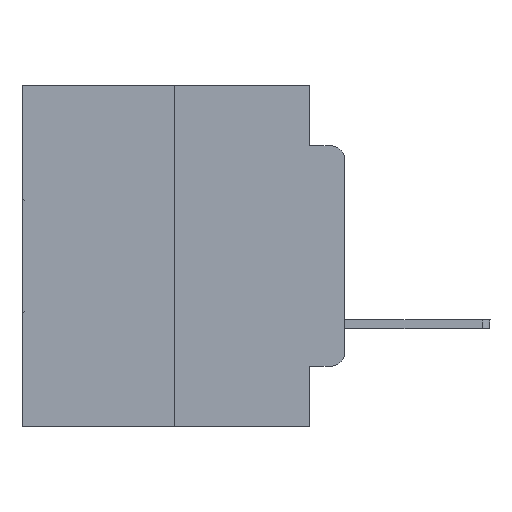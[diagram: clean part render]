
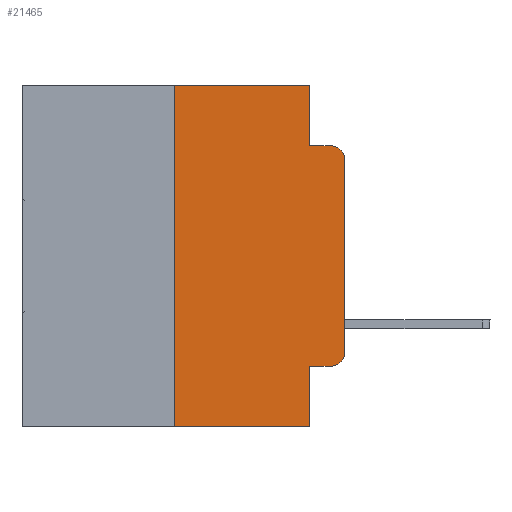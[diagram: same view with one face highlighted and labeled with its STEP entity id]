
A CAD part, left-side view. The second image highlights one B-rep face of the part: STEP entity #21465.
In plain terms, the highlighted planar face has unit normal (-1, 0, 0).
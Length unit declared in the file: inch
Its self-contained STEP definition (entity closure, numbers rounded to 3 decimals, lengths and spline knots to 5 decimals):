
#18 = LINE ( 'NONE', #8646, #12832 ) ;
#384 = CARTESIAN_POINT ( 'NONE',  ( 0., 0.25, -0.5 ) ) ;
#509 = VERTEX_POINT ( 'NONE', #1421 ) ;
#519 = EDGE_CURVE ( 'NONE', #12336, #18329, #22725, .T. ) ;
#858 = ORIENTED_EDGE ( 'NONE', *, *, #20175, .T. ) ;
#1063 = DIRECTION ( 'NONE',  ( -1., 0., 0. ) ) ;
#1421 = CARTESIAN_POINT ( 'NONE',  ( 0., 0.25, 0. ) ) ;
#1689 = VECTOR ( 'NONE', #12039, 39.37008 ) ;
#2119 = EDGE_CURVE ( 'NONE', #12896, #6646, #10922, .T. ) ;
#2352 = VECTOR ( 'NONE', #19069, 39.37008 ) ;
#2732 = CARTESIAN_POINT ( 'NONE',  ( 0., 0.051, -0.4115 ) ) ;
#3836 = VERTEX_POINT ( 'NONE', #13473 ) ;
#4869 = LINE ( 'NONE', #22501, #25134 ) ;
#5114 = AXIS2_PLACEMENT_3D ( 'NONE', #24901, #14475, #14336 ) ;
#5531 = VECTOR ( 'NONE', #14047, 39.37008 ) ;
#5994 = ORIENTED_EDGE ( 'NONE', *, *, #22789, .T. ) ;
#6082 = DIRECTION ( 'NONE',  ( 0., 0., -1. ) ) ;
#6646 = VERTEX_POINT ( 'NONE', #12520 ) ;
#6706 = DIRECTION ( 'NONE',  ( 0., 0., 1. ) ) ;
#7362 = EDGE_CURVE ( 'NONE', #26900, #12896, #23975, .T. ) ;
#7705 = PLANE ( 'NONE',  #5114 ) ;
#7989 = DIRECTION ( 'NONE',  ( 0., 0., -1. ) ) ;
#8122 = EDGE_CURVE ( 'NONE', #6646, #16722, #8678, .T. ) ;
#8245 = AXIS2_PLACEMENT_3D ( 'NONE', #20702, #1063, #7989 ) ;
#8646 = CARTESIAN_POINT ( 'NONE',  ( 0., 0.473, -0.5 ) ) ;
#8678 = CIRCLE ( 'NONE', #8245, 0.02 ) ;
#8717 = VERTEX_POINT ( 'NONE', #13815 ) ;
#9290 = CARTESIAN_POINT ( 'NONE',  ( 0., 0.051, -0.5 ) ) ;
#9889 = DIRECTION ( 'NONE',  ( -1., 0., 0. ) ) ;
#10617 = ORIENTED_EDGE ( 'NONE', *, *, #2119, .T. ) ;
#10922 = LINE ( 'NONE', #13599, #22407 ) ;
#11024 = DIRECTION ( 'NONE',  ( 0., -1., 0. ) ) ;
#11562 = ORIENTED_EDGE ( 'NONE', *, *, #14451, .F. ) ;
#11767 = CARTESIAN_POINT ( 'NONE',  ( 0., 0.25, 0. ) ) ;
#11982 = CARTESIAN_POINT ( 'NONE',  ( 0., 0.02, -0.0885 ) ) ;
#12039 = DIRECTION ( 'NONE',  ( 0., 0., 1. ) ) ;
#12336 = VERTEX_POINT ( 'NONE', #2732 ) ;
#12520 = CARTESIAN_POINT ( 'NONE',  ( 0., 0., -0.1085 ) ) ;
#12832 = VECTOR ( 'NONE', #19106, 39.37008 ) ;
#12896 = VERTEX_POINT ( 'NONE', #20054 ) ;
#13170 = AXIS2_PLACEMENT_3D ( 'NONE', #25533, #9889, #6082 ) ;
#13473 = CARTESIAN_POINT ( 'NONE',  ( 0., 0.051, -0.0885 ) ) ;
#13599 = CARTESIAN_POINT ( 'NONE',  ( 0., 0., 0. ) ) ;
#13815 = CARTESIAN_POINT ( 'NONE',  ( 0., 0.051, 0. ) ) ;
#14047 = DIRECTION ( 'NONE',  ( 0., -1., 0. ) ) ;
#14336 = DIRECTION ( 'NONE',  ( 0., 0., -1. ) ) ;
#14403 = DIRECTION ( 'NONE',  ( 0., -1., 0. ) ) ;
#14451 = EDGE_CURVE ( 'NONE', #8717, #3836, #4869, .T. ) ;
#14475 = DIRECTION ( 'NONE',  ( 1., 0., 0. ) ) ;
#14545 = EDGE_CURVE ( 'NONE', #15682, #509, #18138, .T. ) ;
#14992 = ORIENTED_EDGE ( 'NONE', *, *, #14545, .F. ) ;
#15008 = VECTOR ( 'NONE', #11024, 39.37008 ) ;
#15467 = DIRECTION ( 'NONE',  ( 0., 0., -1. ) ) ;
#15538 = ORIENTED_EDGE ( 'NONE', *, *, #8122, .T. ) ;
#15682 = VERTEX_POINT ( 'NONE', #384 ) ;
#16313 = LINE ( 'NONE', #24895, #5531 ) ;
#16662 = LINE ( 'NONE', #20617, #27791 ) ;
#16722 = VERTEX_POINT ( 'NONE', #11982 ) ;
#17001 = ORIENTED_EDGE ( 'NONE', *, *, #7362, .T. ) ;
#17274 = ORIENTED_EDGE ( 'NONE', *, *, #19019, .F. ) ;
#17455 = EDGE_LOOP ( 'NONE', ( #10617, #15538, #17274, #11562, #22049, #14992, #5994, #24530, #858, #17001 ) ) ;
#17665 = LINE ( 'NONE', #26240, #15008 ) ;
#18138 = LINE ( 'NONE', #11767, #1689 ) ;
#18329 = VERTEX_POINT ( 'NONE', #9290 ) ;
#19019 = EDGE_CURVE ( 'NONE', #3836, #16722, #17665, .T. ) ;
#19069 = DIRECTION ( 'NONE',  ( 0., 0., -1. ) ) ;
#19106 = DIRECTION ( 'NONE',  ( 0., -1., 0. ) ) ;
#20054 = CARTESIAN_POINT ( 'NONE',  ( 0., 0., -0.3915 ) ) ;
#20175 = EDGE_CURVE ( 'NONE', #12336, #26900, #16313, .T. ) ;
#20617 = CARTESIAN_POINT ( 'NONE',  ( 0., 0.473, 0. ) ) ;
#20702 = CARTESIAN_POINT ( 'NONE',  ( 0., 0.02, -0.1085 ) ) ;
#21096 = CARTESIAN_POINT ( 'NONE',  ( 0., 0.02, -0.4115 ) ) ;
#21465 = ADVANCED_FACE ( 'NONE', ( #27018 ), #7705, .F. ) ;
#22049 = ORIENTED_EDGE ( 'NONE', *, *, #26076, .F. ) ;
#22407 = VECTOR ( 'NONE', #6706, 39.37008 ) ;
#22501 = CARTESIAN_POINT ( 'NONE',  ( 0., 0.051, 0. ) ) ;
#22725 = LINE ( 'NONE', #22867, #2352 ) ;
#22789 = EDGE_CURVE ( 'NONE', #15682, #18329, #18, .T. ) ;
#22867 = CARTESIAN_POINT ( 'NONE',  ( 0., 0.051, 0. ) ) ;
#23975 = CIRCLE ( 'NONE', #13170, 0.02 ) ;
#24530 = ORIENTED_EDGE ( 'NONE', *, *, #519, .F. ) ;
#24895 = CARTESIAN_POINT ( 'NONE',  ( 0., 0.051, -0.4115 ) ) ;
#24901 = CARTESIAN_POINT ( 'NONE',  ( 0., 0.473, 0. ) ) ;
#25134 = VECTOR ( 'NONE', #15467, 39.37008 ) ;
#25533 = CARTESIAN_POINT ( 'NONE',  ( 0., 0.02, -0.3915 ) ) ;
#26076 = EDGE_CURVE ( 'NONE', #509, #8717, #16662, .T. ) ;
#26240 = CARTESIAN_POINT ( 'NONE',  ( 0., 0.051, -0.0885 ) ) ;
#26900 = VERTEX_POINT ( 'NONE', #21096 ) ;
#27018 = FACE_OUTER_BOUND ( 'NONE', #17455, .T. ) ;
#27791 = VECTOR ( 'NONE', #14403, 39.37008 ) ;
